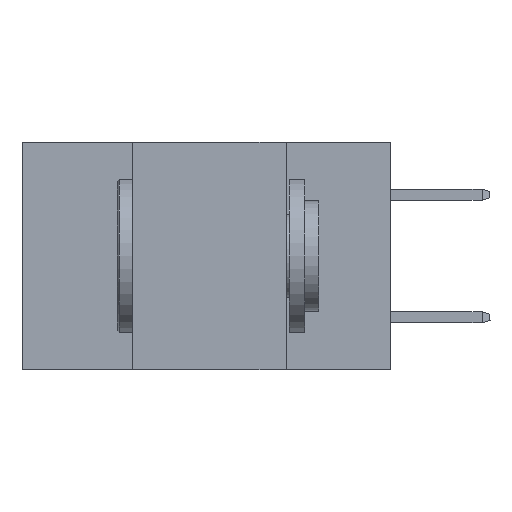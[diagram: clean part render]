
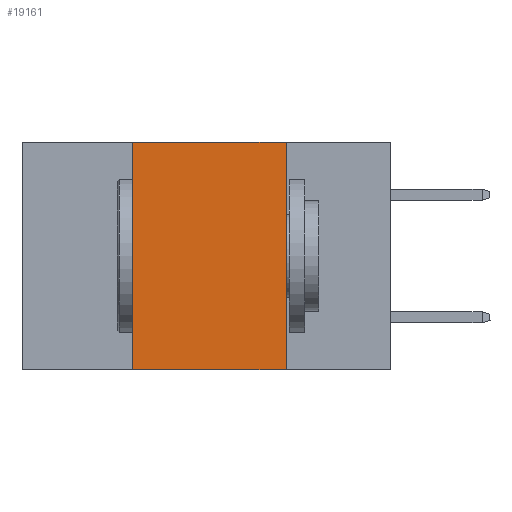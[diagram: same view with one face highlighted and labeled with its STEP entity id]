
A CAD part, left-side view. The second image highlights one B-rep face of the part: STEP entity #19161.
In plain terms, the highlighted planar face has unit normal (-1, 0, 0).
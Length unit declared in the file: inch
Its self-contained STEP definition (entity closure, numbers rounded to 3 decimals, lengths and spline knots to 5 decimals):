
#3120 = VERTEX_POINT ( 'NONE', #28278 ) ;
#5387 = VECTOR ( 'NONE', #34949, 39.37008 ) ;
#5842 = LINE ( 'NONE', #24083, #8798 ) ;
#6176 = VERTEX_POINT ( 'NONE', #9500 ) ;
#8795 = LINE ( 'NONE', #31995, #5387 ) ;
#8798 = VECTOR ( 'NONE', #10570, 39.37008 ) ;
#9500 = CARTESIAN_POINT ( 'NONE',  ( 0., 0.42, 0. ) ) ;
#9660 = ORIENTED_EDGE ( 'NONE', *, *, #30739, .T. ) ;
#10458 = CARTESIAN_POINT ( 'NONE',  ( 0., 0.6, 0. ) ) ;
#10570 = DIRECTION ( 'NONE',  ( 0., 0., 1. ) ) ;
#11594 = LINE ( 'NONE', #31738, #13281 ) ;
#13281 = VECTOR ( 'NONE', #17878, 39.37008 ) ;
#13920 = DIRECTION ( 'NONE',  ( 0., -1., 0. ) ) ;
#14034 = CARTESIAN_POINT ( 'NONE',  ( 0., 0.6, 0. ) ) ;
#14617 = EDGE_CURVE ( 'NONE', #20386, #6176, #5842, .T. ) ;
#15191 = EDGE_LOOP ( 'NONE', ( #28515, #23770, #26165, #9660 ) ) ;
#16051 = EDGE_CURVE ( 'NONE', #6176, #24188, #27775, .T. ) ;
#16220 = CARTESIAN_POINT ( 'NONE',  ( 0., 0.42, -0.37 ) ) ;
#17878 = DIRECTION ( 'NONE',  ( 0., -1., 0. ) ) ;
#19161 = ADVANCED_FACE ( 'NONE', ( #25639 ), #21359, .F. ) ;
#20386 = VERTEX_POINT ( 'NONE', #16220 ) ;
#21359 = PLANE ( 'NONE',  #34307 ) ;
#23770 = ORIENTED_EDGE ( 'NONE', *, *, #16051, .F. ) ;
#24083 = CARTESIAN_POINT ( 'NONE',  ( 0., 0.42, 0. ) ) ;
#24188 = VERTEX_POINT ( 'NONE', #32625 ) ;
#24825 = VECTOR ( 'NONE', #13920, 39.37008 ) ;
#25639 = FACE_OUTER_BOUND ( 'NONE', #15191, .T. ) ;
#26165 = ORIENTED_EDGE ( 'NONE', *, *, #14617, .F. ) ;
#26468 = DIRECTION ( 'NONE',  ( 1., 0., 0. ) ) ;
#27775 = LINE ( 'NONE', #14034, #24825 ) ;
#28278 = CARTESIAN_POINT ( 'NONE',  ( 0., 0.17, -0.37 ) ) ;
#28515 = ORIENTED_EDGE ( 'NONE', *, *, #34906, .F. ) ;
#29204 = DIRECTION ( 'NONE',  ( 0., 0., -1. ) ) ;
#30739 = EDGE_CURVE ( 'NONE', #20386, #3120, #11594, .T. ) ;
#31738 = CARTESIAN_POINT ( 'NONE',  ( 0., 0.6, -0.37 ) ) ;
#31995 = CARTESIAN_POINT ( 'NONE',  ( 0., 0.17, 0. ) ) ;
#32625 = CARTESIAN_POINT ( 'NONE',  ( 0., 0.17, 0. ) ) ;
#34307 = AXIS2_PLACEMENT_3D ( 'NONE', #10458, #26468, #29204 ) ;
#34906 = EDGE_CURVE ( 'NONE', #24188, #3120, #8795, .T. ) ;
#34949 = DIRECTION ( 'NONE',  ( 0., 0., -1. ) ) ;
